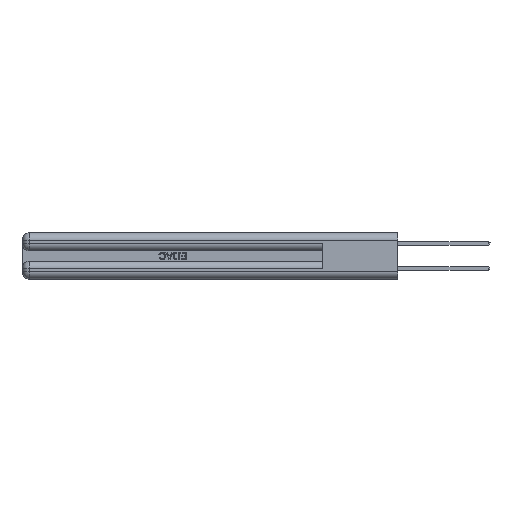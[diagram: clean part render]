
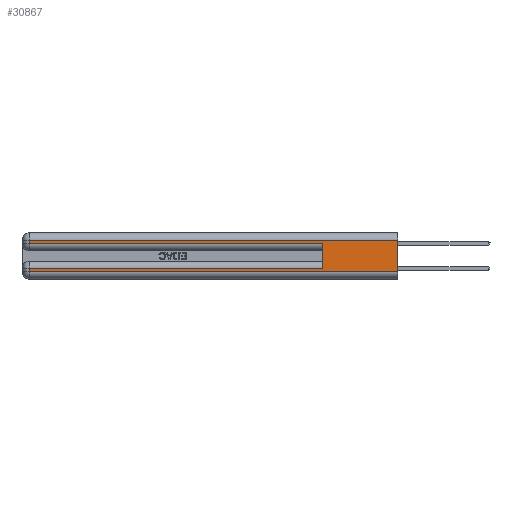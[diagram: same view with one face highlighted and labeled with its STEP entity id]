
A CAD part, left-side view. The second image highlights one B-rep face of the part: STEP entity #30867.
In plain terms, the highlighted planar face has unit normal (-1, 0, 0).
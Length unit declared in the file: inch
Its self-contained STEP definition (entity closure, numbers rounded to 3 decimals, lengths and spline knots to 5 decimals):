
#214 = CARTESIAN_POINT ( 'NONE',  ( 0., 0., 0.37 ) ) ;
#293 = CARTESIAN_POINT ( 'NONE',  ( 0., 2.94, 0.37 ) ) ;
#1305 = CARTESIAN_POINT ( 'NONE',  ( 0., 2.94, 0.06 ) ) ;
#1553 = ORIENTED_EDGE ( 'NONE', *, *, #16719, .T. ) ;
#2628 = VERTEX_POINT ( 'NONE', #1305 ) ;
#3156 = EDGE_CURVE ( 'NONE', #8597, #10577, #25852, .T. ) ;
#3739 = CARTESIAN_POINT ( 'NONE',  ( 0., 0., 0.31 ) ) ;
#4166 = DIRECTION ( 'NONE',  ( 0., 0., -1. ) ) ;
#4659 = EDGE_CURVE ( 'NONE', #29165, #47169, #8796, .T. ) ;
#4679 = CARTESIAN_POINT ( 'NONE',  ( 0., 0., 0.06 ) ) ;
#5225 = CARTESIAN_POINT ( 'NONE',  ( 0., 0.6, 0.145 ) ) ;
#5577 = FACE_OUTER_BOUND ( 'NONE', #14169, .T. ) ;
#5989 = EDGE_CURVE ( 'NONE', #7612, #10853, #36475, .T. ) ;
#6150 = DIRECTION ( 'NONE',  ( 0., -1., 0. ) ) ;
#6620 = CARTESIAN_POINT ( 'NONE',  ( 0., 2.94, 0.285 ) ) ;
#7033 = ORIENTED_EDGE ( 'NONE', *, *, #42364, .T. ) ;
#7612 = VERTEX_POINT ( 'NONE', #6620 ) ;
#8198 = DIRECTION ( 'NONE',  ( 0., 0., -1. ) ) ;
#8597 = VERTEX_POINT ( 'NONE', #32406 ) ;
#8796 = LINE ( 'NONE', #41514, #47326 ) ;
#10577 = VERTEX_POINT ( 'NONE', #4679 ) ;
#10853 = VERTEX_POINT ( 'NONE', #33902 ) ;
#11113 = LINE ( 'NONE', #41244, #18964 ) ;
#11550 = CARTESIAN_POINT ( 'NONE',  ( 0., 2.94, 0.31 ) ) ;
#11873 = DIRECTION ( 'NONE',  ( 1., 0., 0. ) ) ;
#12437 = LINE ( 'NONE', #5225, #41975 ) ;
#12512 = LINE ( 'NONE', #29319, #31893 ) ;
#12543 = VECTOR ( 'NONE', #4166, 39.37008 ) ;
#12793 = EDGE_CURVE ( 'NONE', #30132, #7612, #11113, .T. ) ;
#13681 = ORIENTED_EDGE ( 'NONE', *, *, #4659, .T. ) ;
#13770 = LINE ( 'NONE', #293, #12543 ) ;
#14169 = EDGE_LOOP ( 'NONE', ( #18476, #1553, #22116, #36018, #26970, #13681, #23944, #7033 ) ) ;
#16719 = EDGE_CURVE ( 'NONE', #8597, #30132, #30672, .T. ) ;
#18476 = ORIENTED_EDGE ( 'NONE', *, *, #3156, .F. ) ;
#18851 = EDGE_CURVE ( 'NONE', #47169, #2628, #13770, .T. ) ;
#18964 = VECTOR ( 'NONE', #29860, 39.37008 ) ;
#22116 = ORIENTED_EDGE ( 'NONE', *, *, #12793, .T. ) ;
#22335 = DIRECTION ( 'NONE',  ( 0., 1., 0. ) ) ;
#23393 = CARTESIAN_POINT ( 'NONE',  ( 0., 0., 0.285 ) ) ;
#23740 = AXIS2_PLACEMENT_3D ( 'NONE', #214, #11873, #38843 ) ;
#23944 = ORIENTED_EDGE ( 'NONE', *, *, #18851, .T. ) ;
#24456 = DIRECTION ( 'NONE',  ( 0., 0., 1. ) ) ;
#25852 = LINE ( 'NONE', #39051, #36128 ) ;
#26117 = CARTESIAN_POINT ( 'NONE',  ( 0., 2.94, 0.085 ) ) ;
#26910 = DIRECTION ( 'NONE',  ( 0., 1., 0. ) ) ;
#26970 = ORIENTED_EDGE ( 'NONE', *, *, #41504, .F. ) ;
#29165 = VERTEX_POINT ( 'NONE', #36139 ) ;
#29319 = CARTESIAN_POINT ( 'NONE',  ( 0., 0., 0.06 ) ) ;
#29860 = DIRECTION ( 'NONE',  ( 0., 0., -1. ) ) ;
#30132 = VERTEX_POINT ( 'NONE', #11550 ) ;
#30672 = LINE ( 'NONE', #3739, #38451 ) ;
#30867 = ADVANCED_FACE ( 'NONE', ( #5577 ), #35017, .F. ) ;
#31360 = DIRECTION ( 'NONE',  ( 0., -1., 0. ) ) ;
#31660 = VECTOR ( 'NONE', #31360, 39.37008 ) ;
#31893 = VECTOR ( 'NONE', #6150, 39.37008 ) ;
#32406 = CARTESIAN_POINT ( 'NONE',  ( 0., 0., 0.31 ) ) ;
#33902 = CARTESIAN_POINT ( 'NONE',  ( 0., 0.6, 0.285 ) ) ;
#35017 = PLANE ( 'NONE',  #23740 ) ;
#36018 = ORIENTED_EDGE ( 'NONE', *, *, #5989, .T. ) ;
#36128 = VECTOR ( 'NONE', #8198, 39.37008 ) ;
#36139 = CARTESIAN_POINT ( 'NONE',  ( 0., 0.6, 0.085 ) ) ;
#36475 = LINE ( 'NONE', #23393, #31660 ) ;
#38451 = VECTOR ( 'NONE', #26910, 39.37008 ) ;
#38843 = DIRECTION ( 'NONE',  ( 0., 0., -1. ) ) ;
#39051 = CARTESIAN_POINT ( 'NONE',  ( 0., 0., 0.37 ) ) ;
#41244 = CARTESIAN_POINT ( 'NONE',  ( 0., 2.94, 0.37 ) ) ;
#41504 = EDGE_CURVE ( 'NONE', #29165, #10853, #12437, .T. ) ;
#41514 = CARTESIAN_POINT ( 'NONE',  ( 0., 0., 0.085 ) ) ;
#41975 = VECTOR ( 'NONE', #24456, 39.37008 ) ;
#42364 = EDGE_CURVE ( 'NONE', #2628, #10577, #12512, .T. ) ;
#47169 = VERTEX_POINT ( 'NONE', #26117 ) ;
#47326 = VECTOR ( 'NONE', #22335, 39.37008 ) ;
